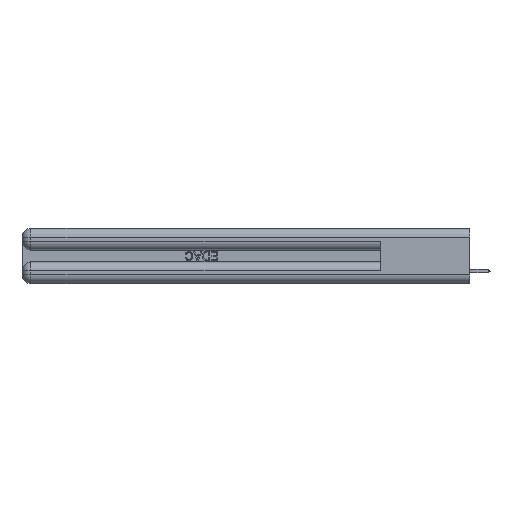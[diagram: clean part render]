
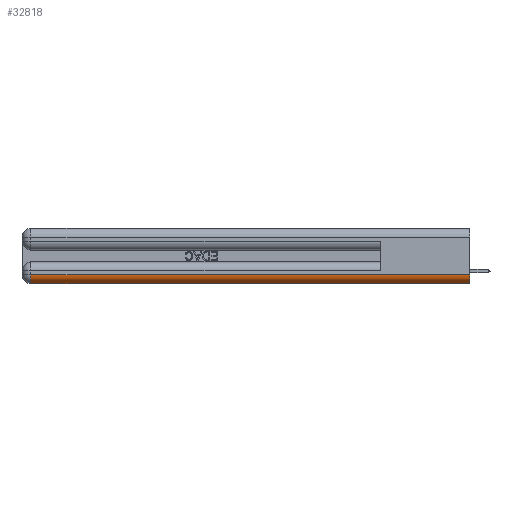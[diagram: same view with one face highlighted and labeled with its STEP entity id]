
A CAD part, left-side view. The second image highlights one B-rep face of the part: STEP entity #32818.
In plain terms, the highlighted cylindrical face has radius 1.524 mm (diameter 3.048 mm), a partial arc.
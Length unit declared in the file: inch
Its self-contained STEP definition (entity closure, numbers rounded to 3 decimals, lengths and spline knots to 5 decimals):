
#69 = LINE ( 'NONE', #31771, #4104 ) ;
#255 = ORIENTED_EDGE ( 'NONE', *, *, #30231, .F. ) ;
#618 = CARTESIAN_POINT ( 'NONE',  ( 0., 2.94, 0.06 ) ) ;
#865 = CARTESIAN_POINT ( 'NONE',  ( 0.06, 2.94, 0. ) ) ;
#2513 = VERTEX_POINT ( 'NONE', #9828 ) ;
#2743 = CIRCLE ( 'NONE', #7715, 0.06 ) ;
#4104 = VECTOR ( 'NONE', #34875, 39.37008 ) ;
#5283 = EDGE_CURVE ( 'NONE', #17809, #37876, #28289, .T. ) ;
#7715 = AXIS2_PLACEMENT_3D ( 'NONE', #17072, #20009, #20560 ) ;
#8323 = DIRECTION ( 'NONE',  ( 0., -1., 0. ) ) ;
#9828 = CARTESIAN_POINT ( 'NONE',  ( 0.06, 0., 0. ) ) ;
#10597 = DIRECTION ( 'NONE',  ( 0., 1., 0. ) ) ;
#11798 = CARTESIAN_POINT ( 'NONE',  ( 0., 0., 0.06 ) ) ;
#14521 = EDGE_LOOP ( 'NONE', ( #255, #17769, #16521, #39359 ) ) ;
#15043 = CARTESIAN_POINT ( 'NONE',  ( 0., 0., 0.06 ) ) ;
#16521 = ORIENTED_EDGE ( 'NONE', *, *, #27158, .F. ) ;
#17072 = CARTESIAN_POINT ( 'NONE',  ( 0.06, 2.94, 0.06 ) ) ;
#17117 = CARTESIAN_POINT ( 'NONE',  ( 0.06, 0., 0.06 ) ) ;
#17769 = ORIENTED_EDGE ( 'NONE', *, *, #5283, .F. ) ;
#17809 = VERTEX_POINT ( 'NONE', #618 ) ;
#20009 = DIRECTION ( 'NONE',  ( 0., 1., 0. ) ) ;
#20560 = DIRECTION ( 'NONE',  ( 0., 0., 1. ) ) ;
#23841 = CYLINDRICAL_SURFACE ( 'NONE', #31986, 0.06 ) ;
#24459 = AXIS2_PLACEMENT_3D ( 'NONE', #17117, #36868, #38121 ) ;
#27158 = EDGE_CURVE ( 'NONE', #34140, #17809, #2743, .T. ) ;
#28289 = LINE ( 'NONE', #11798, #39291 ) ;
#30231 = EDGE_CURVE ( 'NONE', #37876, #2513, #31247, .T. ) ;
#31247 = CIRCLE ( 'NONE', #24459, 0.06 ) ;
#31771 = CARTESIAN_POINT ( 'NONE',  ( 0.06, 3., 0. ) ) ;
#31986 = AXIS2_PLACEMENT_3D ( 'NONE', #36198, #10597, #39583 ) ;
#32818 = ADVANCED_FACE ( 'NONE', ( #39520 ), #23841, .T. ) ;
#34140 = VERTEX_POINT ( 'NONE', #865 ) ;
#34875 = DIRECTION ( 'NONE',  ( 0., 1., 0. ) ) ;
#36198 = CARTESIAN_POINT ( 'NONE',  ( 0.06, 0., 0.06 ) ) ;
#36868 = DIRECTION ( 'NONE',  ( 0., -1., 0. ) ) ;
#37876 = VERTEX_POINT ( 'NONE', #15043 ) ;
#38121 = DIRECTION ( 'NONE',  ( 0., 0., 1. ) ) ;
#39291 = VECTOR ( 'NONE', #8323, 39.37008 ) ;
#39359 = ORIENTED_EDGE ( 'NONE', *, *, #40836, .F. ) ;
#39520 = FACE_OUTER_BOUND ( 'NONE', #14521, .T. ) ;
#39583 = DIRECTION ( 'NONE',  ( 0., 0., 1. ) ) ;
#40836 = EDGE_CURVE ( 'NONE', #2513, #34140, #69, .T. ) ;
